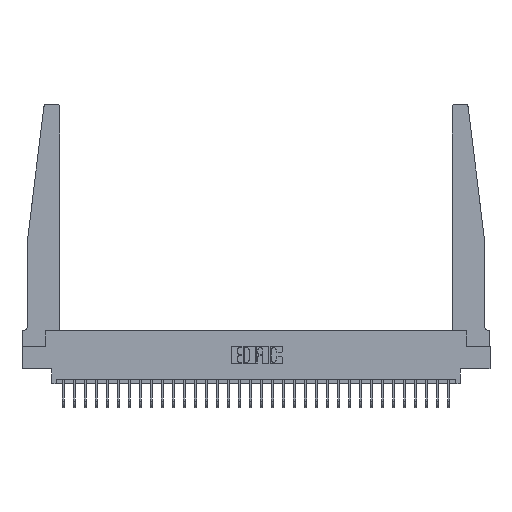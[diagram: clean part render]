
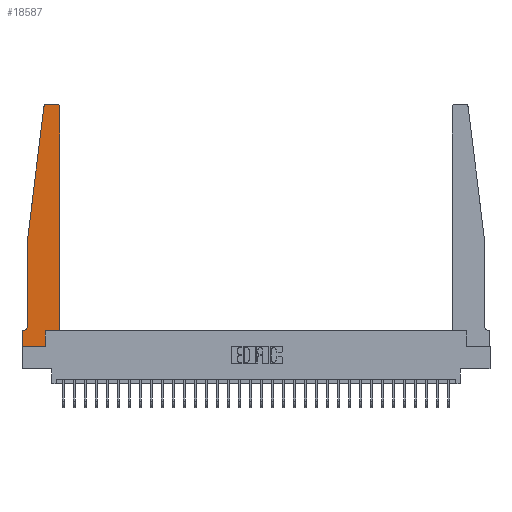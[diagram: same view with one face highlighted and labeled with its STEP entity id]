
A CAD part, top view. The second image highlights one B-rep face of the part: STEP entity #18587.
In plain terms, the highlighted planar face has unit normal (0, 0, 1).
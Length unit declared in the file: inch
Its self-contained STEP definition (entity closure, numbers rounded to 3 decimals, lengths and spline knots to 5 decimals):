
#210 = VERTEX_POINT ( 'NONE', #3190 ) ;
#222 = VECTOR ( 'NONE', #13109, 39.37008 ) ;
#249 = DIRECTION ( 'NONE',  ( 0., 0., 1. ) ) ;
#1754 = AXIS2_PLACEMENT_3D ( 'NONE', #3568, #27946, #6436 ) ;
#2039 = AXIS2_PLACEMENT_3D ( 'NONE', #12983, #8423, #4455 ) ;
#2053 = LINE ( 'NONE', #21035, #22620 ) ;
#2119 = DIRECTION ( 'NONE',  ( -1., 0., 0. ) ) ;
#2237 = CARTESIAN_POINT ( 'NONE',  ( 0.065, 0.2375, 0.37 ) ) ;
#2288 = EDGE_CURVE ( 'NONE', #3720, #2363, #2053, .T. ) ;
#2291 = VERTEX_POINT ( 'NONE', #2237 ) ;
#2363 = VERTEX_POINT ( 'NONE', #19134 ) ;
#2436 = ORIENTED_EDGE ( 'NONE', *, *, #20363, .T. ) ;
#2785 = CARTESIAN_POINT ( 'NONE',  ( 0., 0.1875, 0.37 ) ) ;
#3190 = CARTESIAN_POINT ( 'NONE',  ( 0., 0., 0.37 ) ) ;
#3255 = ORIENTED_EDGE ( 'NONE', *, *, #3921, .T. ) ;
#3326 = LINE ( 'NONE', #4721, #28038 ) ;
#3331 = LINE ( 'NONE', #9829, #10138 ) ;
#3568 = CARTESIAN_POINT ( 'NONE',  ( 0.27653, 2.72, 0.37 ) ) ;
#3720 = VERTEX_POINT ( 'NONE', #25173 ) ;
#3921 = EDGE_CURVE ( 'NONE', #2363, #7355, #14677, .T. ) ;
#4298 = VERTEX_POINT ( 'NONE', #11829 ) ;
#4420 = VECTOR ( 'NONE', #16884, 39.37008 ) ;
#4455 = DIRECTION ( 'NONE',  ( 1., 0., 0. ) ) ;
#4664 = EDGE_CURVE ( 'NONE', #8044, #13533, #10814, .T. ) ;
#4687 = ORIENTED_EDGE ( 'NONE', *, *, #18316, .T. ) ;
#4721 = CARTESIAN_POINT ( 'NONE',  ( 0.065, 1.25, 0.37 ) ) ;
#5292 = ORIENTED_EDGE ( 'NONE', *, *, #14313, .T. ) ;
#5351 = VECTOR ( 'NONE', #20086, 39.37008 ) ;
#6436 = DIRECTION ( 'NONE',  ( 1., 0., 0. ) ) ;
#7208 = CARTESIAN_POINT ( 'NONE',  ( 0.425, 0.18, 0.37 ) ) ;
#7355 = VERTEX_POINT ( 'NONE', #18572 ) ;
#7571 = EDGE_CURVE ( 'NONE', #2291, #4298, #19541, .T. ) ;
#7734 = CARTESIAN_POINT ( 'NONE',  ( 0., 0.1875, 0.37 ) ) ;
#8031 = EDGE_CURVE ( 'NONE', #28172, #3720, #27804, .T. ) ;
#8044 = VERTEX_POINT ( 'NONE', #23483 ) ;
#8423 = DIRECTION ( 'NONE',  ( 0., 0., 1. ) ) ;
#8784 = VECTOR ( 'NONE', #15644, 39.37008 ) ;
#8874 = EDGE_CURVE ( 'NONE', #15670, #8044, #25920, .T. ) ;
#9829 = CARTESIAN_POINT ( 'NONE',  ( 0., 0., 0.37 ) ) ;
#9950 = PLANE ( 'NONE',  #10594 ) ;
#10138 = VECTOR ( 'NONE', #26403, 39.37008 ) ;
#10594 = AXIS2_PLACEMENT_3D ( 'NONE', #2785, #249, #14810 ) ;
#10627 = ORIENTED_EDGE ( 'NONE', *, *, #2288, .T. ) ;
#10814 = LINE ( 'NONE', #11404, #4420 ) ;
#11404 = CARTESIAN_POINT ( 'NONE',  ( 0.425, 0.18, 0.37 ) ) ;
#11527 = ORIENTED_EDGE ( 'NONE', *, *, #4664, .T. ) ;
#11829 = CARTESIAN_POINT ( 'NONE',  ( 0.015, 0.1875, 0.37 ) ) ;
#12108 = DIRECTION ( 'NONE',  ( 0., 1., 0. ) ) ;
#12400 = EDGE_CURVE ( 'NONE', #4298, #23561, #22253, .T. ) ;
#12983 = CARTESIAN_POINT ( 'NONE',  ( 0.395, 2.72, 0.37 ) ) ;
#13074 = CARTESIAN_POINT ( 'NONE',  ( 0.065, 0.1875, 0.37 ) ) ;
#13109 = DIRECTION ( 'NONE',  ( -0.122, -0.992, 0. ) ) ;
#13533 = VERTEX_POINT ( 'NONE', #15222 ) ;
#14313 = EDGE_CURVE ( 'NONE', #23561, #210, #19539, .T. ) ;
#14360 = DIRECTION ( 'NONE',  ( 0., -1., 0. ) ) ;
#14677 = CIRCLE ( 'NONE', #1754, 0.03 ) ;
#14810 = DIRECTION ( 'NONE',  ( 1., 0., 0. ) ) ;
#15222 = CARTESIAN_POINT ( 'NONE',  ( 0.425, 0.18, 0.37 ) ) ;
#15644 = DIRECTION ( 'NONE',  ( 0., 1., 0. ) ) ;
#15670 = VERTEX_POINT ( 'NONE', #27159 ) ;
#16400 = LINE ( 'NONE', #7208, #27237 ) ;
#16412 = EDGE_CURVE ( 'NONE', #210, #15670, #3331, .T. ) ;
#16816 = ORIENTED_EDGE ( 'NONE', *, *, #8031, .T. ) ;
#16853 = FACE_OUTER_BOUND ( 'NONE', #21720, .T. ) ;
#16884 = DIRECTION ( 'NONE',  ( 1., 0., 0. ) ) ;
#17315 = DIRECTION ( 'NONE',  ( -1., 0., 0. ) ) ;
#17513 = DIRECTION ( 'NONE',  ( 0., 0., -1. ) ) ;
#17846 = DIRECTION ( 'NONE',  ( -1., 0., 0. ) ) ;
#18316 = EDGE_CURVE ( 'NONE', #7355, #30616, #22694, .T. ) ;
#18572 = CARTESIAN_POINT ( 'NONE',  ( 0.24675, 2.72367, 0.37 ) ) ;
#18587 = ADVANCED_FACE ( 'NONE', ( #16853 ), #9950, .T. ) ;
#18921 = CARTESIAN_POINT ( 'NONE',  ( 0.065, 1.25, 0.37 ) ) ;
#19134 = CARTESIAN_POINT ( 'NONE',  ( 0.27653, 2.75, 0.37 ) ) ;
#19539 = LINE ( 'NONE', #24808, #5351 ) ;
#19541 = CIRCLE ( 'NONE', #19842, 0.05 ) ;
#19842 = AXIS2_PLACEMENT_3D ( 'NONE', #26854, #17513, #17315 ) ;
#20086 = DIRECTION ( 'NONE',  ( 0., -1., 0. ) ) ;
#20317 = CARTESIAN_POINT ( 'NONE',  ( 0.2605, 0.18, 0.37 ) ) ;
#20348 = VECTOR ( 'NONE', #17846, 39.37008 ) ;
#20363 = EDGE_CURVE ( 'NONE', #30616, #2291, #3326, .T. ) ;
#20578 = ORIENTED_EDGE ( 'NONE', *, *, #12400, .T. ) ;
#21035 = CARTESIAN_POINT ( 'NONE',  ( 0.25, 2.75, 0.37 ) ) ;
#21720 = EDGE_LOOP ( 'NONE', ( #10627, #3255, #4687, #2436, #27718, #20578, #5292, #27969, #25284, #11527, #27303, #16816 ) ) ;
#22253 = LINE ( 'NONE', #13074, #20348 ) ;
#22620 = VECTOR ( 'NONE', #2119, 39.37008 ) ;
#22694 = LINE ( 'NONE', #24993, #222 ) ;
#23483 = CARTESIAN_POINT ( 'NONE',  ( 0.2605, 0.18, 0.37 ) ) ;
#23561 = VERTEX_POINT ( 'NONE', #7734 ) ;
#24808 = CARTESIAN_POINT ( 'NONE',  ( 0., 0., 0.37 ) ) ;
#24993 = CARTESIAN_POINT ( 'NONE',  ( 0.065, 1.25, 0.37 ) ) ;
#25173 = CARTESIAN_POINT ( 'NONE',  ( 0.395, 2.75, 0.37 ) ) ;
#25284 = ORIENTED_EDGE ( 'NONE', *, *, #8874, .T. ) ;
#25920 = LINE ( 'NONE', #20317, #8784 ) ;
#26403 = DIRECTION ( 'NONE',  ( 1., 0., 0. ) ) ;
#26854 = CARTESIAN_POINT ( 'NONE',  ( 0.015, 0.2375, 0.37 ) ) ;
#27159 = CARTESIAN_POINT ( 'NONE',  ( 0.2605, 0., 0.37 ) ) ;
#27237 = VECTOR ( 'NONE', #12108, 39.37008 ) ;
#27303 = ORIENTED_EDGE ( 'NONE', *, *, #29936, .T. ) ;
#27718 = ORIENTED_EDGE ( 'NONE', *, *, #7571, .T. ) ;
#27804 = CIRCLE ( 'NONE', #2039, 0.03 ) ;
#27946 = DIRECTION ( 'NONE',  ( 0., 0., 1. ) ) ;
#27969 = ORIENTED_EDGE ( 'NONE', *, *, #16412, .T. ) ;
#28038 = VECTOR ( 'NONE', #14360, 39.37008 ) ;
#28172 = VERTEX_POINT ( 'NONE', #30085 ) ;
#29936 = EDGE_CURVE ( 'NONE', #13533, #28172, #16400, .T. ) ;
#30085 = CARTESIAN_POINT ( 'NONE',  ( 0.425, 2.72, 0.37 ) ) ;
#30616 = VERTEX_POINT ( 'NONE', #18921 ) ;
